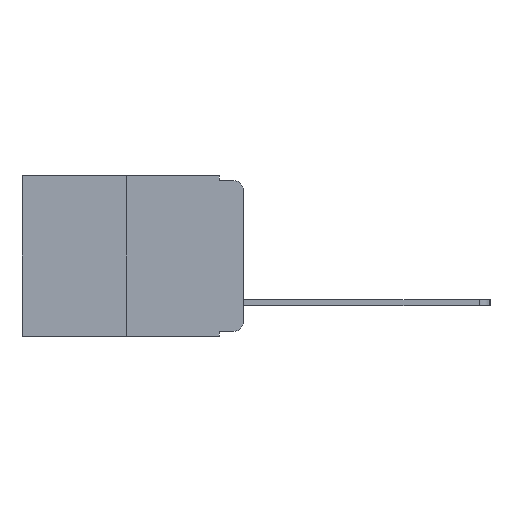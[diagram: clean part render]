
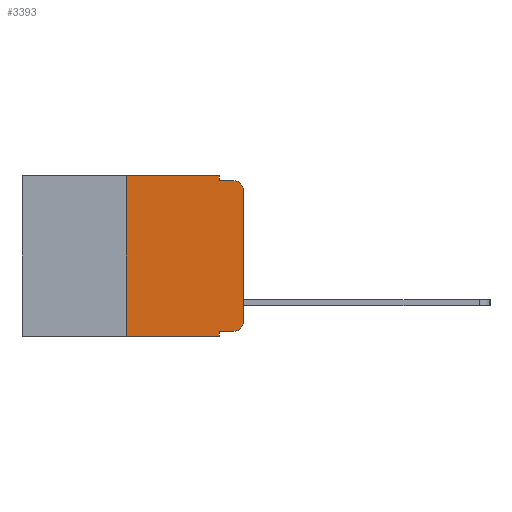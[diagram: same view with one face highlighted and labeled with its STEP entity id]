
A CAD part, left-side view. The second image highlights one B-rep face of the part: STEP entity #3393.
In plain terms, the highlighted planar face has unit normal (-1, 0, 0).
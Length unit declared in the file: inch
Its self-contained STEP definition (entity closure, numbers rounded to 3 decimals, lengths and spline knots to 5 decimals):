
#48 = CARTESIAN_POINT ( 'NONE',  ( 0., 0.051, -0.01 ) ) ;
#77 = CARTESIAN_POINT ( 'NONE',  ( 0., 0.02, -0.313 ) ) ;
#161 = ORIENTED_EDGE ( 'NONE', *, *, #5607, .T. ) ;
#201 = DIRECTION ( 'NONE',  ( 0., -1., 0. ) ) ;
#289 = LINE ( 'NONE', #4228, #5322 ) ;
#311 = EDGE_CURVE ( 'NONE', #5581, #5487, #2353, .T. ) ;
#337 = VERTEX_POINT ( 'NONE', #8537 ) ;
#402 = LINE ( 'NONE', #9976, #2369 ) ;
#940 = VERTEX_POINT ( 'NONE', #2020 ) ;
#942 = CARTESIAN_POINT ( 'NONE',  ( 0., 0., -0.313 ) ) ;
#1115 = CARTESIAN_POINT ( 'NONE',  ( 0., 0.473, 0. ) ) ;
#1177 = CARTESIAN_POINT ( 'NONE',  ( 0., 0.473, -0.343 ) ) ;
#1607 = EDGE_CURVE ( 'NONE', #2757, #5581, #11183, .T. ) ;
#2020 = CARTESIAN_POINT ( 'NONE',  ( 0., 0.02, -0.333 ) ) ;
#2353 = CIRCLE ( 'NONE', #3754, 0.02 ) ;
#2369 = VECTOR ( 'NONE', #3162, 39.37008 ) ;
#2459 = VERTEX_POINT ( 'NONE', #9592 ) ;
#2757 = VERTEX_POINT ( 'NONE', #942 ) ;
#2800 = VERTEX_POINT ( 'NONE', #11131 ) ;
#2861 = EDGE_LOOP ( 'NONE', ( #7321, #9501, #5331, #5614, #3761, #6144, #4033, #11030, #4926, #161 ) ) ;
#2880 = DIRECTION ( 'NONE',  ( 0., 0., -1. ) ) ;
#3162 = DIRECTION ( 'NONE',  ( 0., 0., 1. ) ) ;
#3167 = VECTOR ( 'NONE', #9118, 39.37008 ) ;
#3393 = ADVANCED_FACE ( 'NONE', ( #7858 ), #7482, .F. ) ;
#3419 = VECTOR ( 'NONE', #2880, 39.37008 ) ;
#3452 = CARTESIAN_POINT ( 'NONE',  ( 0., 0.25, -0.343 ) ) ;
#3530 = VERTEX_POINT ( 'NONE', #8083 ) ;
#3754 = AXIS2_PLACEMENT_3D ( 'NONE', #9198, #9171, #9162 ) ;
#3761 = ORIENTED_EDGE ( 'NONE', *, *, #7771, .F. ) ;
#3795 = DIRECTION ( 'NONE',  ( 0., -1., 0. ) ) ;
#3863 = VECTOR ( 'NONE', #3795, 39.37008 ) ;
#4033 = ORIENTED_EDGE ( 'NONE', *, *, #11261, .T. ) ;
#4068 = VERTEX_POINT ( 'NONE', #4292 ) ;
#4084 = VECTOR ( 'NONE', #5679, 39.37008 ) ;
#4228 = CARTESIAN_POINT ( 'NONE',  ( 0., 0.051, -0.333 ) ) ;
#4232 = DIRECTION ( 'NONE',  ( 0., -1., 0. ) ) ;
#4292 = CARTESIAN_POINT ( 'NONE',  ( 0., 0.25, 0. ) ) ;
#4512 = VECTOR ( 'NONE', #8419, 39.37008 ) ;
#4926 = ORIENTED_EDGE ( 'NONE', *, *, #6715, .T. ) ;
#5310 = DIRECTION ( 'NONE',  ( 0., 0., -1. ) ) ;
#5322 = VECTOR ( 'NONE', #4232, 39.37008 ) ;
#5331 = ORIENTED_EDGE ( 'NONE', *, *, #11128, .F. ) ;
#5375 = LINE ( 'NONE', #1177, #7368 ) ;
#5433 = DIRECTION ( 'NONE',  ( -1., 0., 0. ) ) ;
#5487 = VERTEX_POINT ( 'NONE', #6960 ) ;
#5581 = VERTEX_POINT ( 'NONE', #9347 ) ;
#5586 = LINE ( 'NONE', #5722, #3167 ) ;
#5607 = EDGE_CURVE ( 'NONE', #940, #2757, #8542, .T. ) ;
#5614 = ORIENTED_EDGE ( 'NONE', *, *, #8986, .F. ) ;
#5679 = DIRECTION ( 'NONE',  ( 0., -1., 0. ) ) ;
#5722 = CARTESIAN_POINT ( 'NONE',  ( 0., 0.051, 0. ) ) ;
#6144 = ORIENTED_EDGE ( 'NONE', *, *, #7873, .F. ) ;
#6715 = EDGE_CURVE ( 'NONE', #3530, #940, #289, .T. ) ;
#6960 = CARTESIAN_POINT ( 'NONE',  ( 0., 0.02, -0.01 ) ) ;
#7135 = DIRECTION ( 'NONE',  ( 0., 0., -1. ) ) ;
#7295 = EDGE_CURVE ( 'NONE', #3530, #337, #5586, .T. ) ;
#7321 = ORIENTED_EDGE ( 'NONE', *, *, #1607, .T. ) ;
#7368 = VECTOR ( 'NONE', #201, 39.37008 ) ;
#7482 = PLANE ( 'NONE',  #8253 ) ;
#7542 = CARTESIAN_POINT ( 'NONE',  ( 0., 0., 0. ) ) ;
#7771 = EDGE_CURVE ( 'NONE', #4068, #2459, #10613, .T. ) ;
#7858 = FACE_OUTER_BOUND ( 'NONE', #2861, .T. ) ;
#7873 = EDGE_CURVE ( 'NONE', #10932, #4068, #402, .T. ) ;
#8083 = CARTESIAN_POINT ( 'NONE',  ( 0., 0.051, -0.333 ) ) ;
#8253 = AXIS2_PLACEMENT_3D ( 'NONE', #1115, #9120, #7135 ) ;
#8419 = DIRECTION ( 'NONE',  ( 0., 0., 1. ) ) ;
#8450 = LINE ( 'NONE', #48, #4084 ) ;
#8537 = CARTESIAN_POINT ( 'NONE',  ( 0., 0.051, -0.343 ) ) ;
#8542 = CIRCLE ( 'NONE', #9221, 0.02 ) ;
#8986 = EDGE_CURVE ( 'NONE', #2459, #2800, #10190, .T. ) ;
#9118 = DIRECTION ( 'NONE',  ( 0., 0., -1. ) ) ;
#9120 = DIRECTION ( 'NONE',  ( 1., 0., 0. ) ) ;
#9162 = DIRECTION ( 'NONE',  ( 0., 0., -1. ) ) ;
#9171 = DIRECTION ( 'NONE',  ( -1., 0., 0. ) ) ;
#9198 = CARTESIAN_POINT ( 'NONE',  ( 0., 0.02, -0.03 ) ) ;
#9221 = AXIS2_PLACEMENT_3D ( 'NONE', #77, #5433, #5310 ) ;
#9347 = CARTESIAN_POINT ( 'NONE',  ( 0., 0., -0.03 ) ) ;
#9501 = ORIENTED_EDGE ( 'NONE', *, *, #311, .T. ) ;
#9592 = CARTESIAN_POINT ( 'NONE',  ( 0., 0.051, 0. ) ) ;
#9976 = CARTESIAN_POINT ( 'NONE',  ( 0., 0.25, 0. ) ) ;
#10190 = LINE ( 'NONE', #10589, #3419 ) ;
#10589 = CARTESIAN_POINT ( 'NONE',  ( 0., 0.051, 0. ) ) ;
#10613 = LINE ( 'NONE', #11343, #3863 ) ;
#10932 = VERTEX_POINT ( 'NONE', #3452 ) ;
#11030 = ORIENTED_EDGE ( 'NONE', *, *, #7295, .F. ) ;
#11128 = EDGE_CURVE ( 'NONE', #2800, #5487, #8450, .T. ) ;
#11131 = CARTESIAN_POINT ( 'NONE',  ( 0., 0.051, -0.01 ) ) ;
#11183 = LINE ( 'NONE', #7542, #4512 ) ;
#11261 = EDGE_CURVE ( 'NONE', #10932, #337, #5375, .T. ) ;
#11343 = CARTESIAN_POINT ( 'NONE',  ( 0., 0.473, 0. ) ) ;
